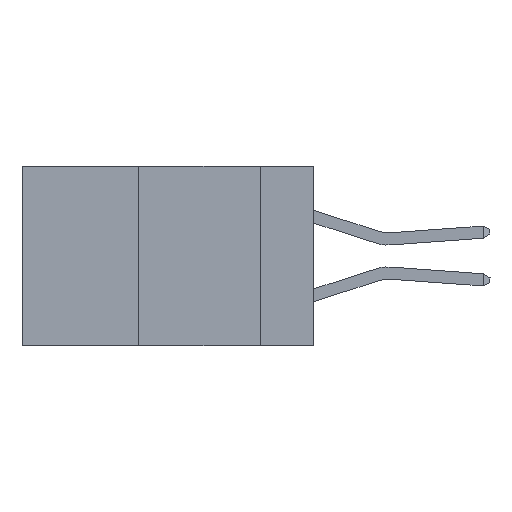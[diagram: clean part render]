
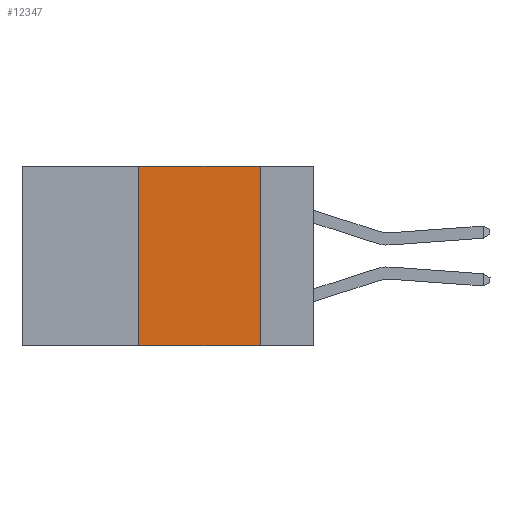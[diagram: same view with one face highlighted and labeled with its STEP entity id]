
A CAD part, left-side view. The second image highlights one B-rep face of the part: STEP entity #12347.
In plain terms, the highlighted planar face has unit normal (-1, 0, 0).
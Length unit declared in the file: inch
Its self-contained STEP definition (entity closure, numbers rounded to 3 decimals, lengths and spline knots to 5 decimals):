
#113 = DIRECTION ( 'NONE',  ( 0., 0., -1. ) ) ;
#137 = LINE ( 'NONE', #12398, #3950 ) ;
#173 = ORIENTED_EDGE ( 'NONE', *, *, #17233, .T. ) ;
#1226 = ORIENTED_EDGE ( 'NONE', *, *, #10822, .F. ) ;
#2858 = EDGE_LOOP ( 'NONE', ( #1226, #11848, #3285, #173 ) ) ;
#3285 = ORIENTED_EDGE ( 'NONE', *, *, #15034, .F. ) ;
#3747 = CARTESIAN_POINT ( 'NONE',  ( 0., 0.11, -0.37 ) ) ;
#3950 = VECTOR ( 'NONE', #15524, 39.37008 ) ;
#5237 = DIRECTION ( 'NONE',  ( 0., 0., 1. ) ) ;
#5273 = VERTEX_POINT ( 'NONE', #16228 ) ;
#5335 = VERTEX_POINT ( 'NONE', #11911 ) ;
#5646 = LINE ( 'NONE', #10524, #16521 ) ;
#5786 = DIRECTION ( 'NONE',  ( 0., 0., -1. ) ) ;
#6332 = VERTEX_POINT ( 'NONE', #3747 ) ;
#7597 = CARTESIAN_POINT ( 'NONE',  ( 0., 0.6, 0. ) ) ;
#9535 = LINE ( 'NONE', #7597, #13103 ) ;
#9648 = EDGE_CURVE ( 'NONE', #5273, #5335, #9535, .T. ) ;
#10524 = CARTESIAN_POINT ( 'NONE',  ( 0., 0.11, 0. ) ) ;
#10822 = EDGE_CURVE ( 'NONE', #5335, #6332, #5646, .T. ) ;
#11848 = ORIENTED_EDGE ( 'NONE', *, *, #9648, .F. ) ;
#11911 = CARTESIAN_POINT ( 'NONE',  ( 0., 0.11, 0. ) ) ;
#12039 = DIRECTION ( 'NONE',  ( 0., -1., 0. ) ) ;
#12243 = CARTESIAN_POINT ( 'NONE',  ( 0., 0.36, -0.37 ) ) ;
#12347 = ADVANCED_FACE ( 'NONE', ( #13664 ), #13435, .F. ) ;
#12398 = CARTESIAN_POINT ( 'NONE',  ( 0., 0.6, -0.37 ) ) ;
#13103 = VECTOR ( 'NONE', #12039, 39.37008 ) ;
#13435 = PLANE ( 'NONE',  #16204 ) ;
#13664 = FACE_OUTER_BOUND ( 'NONE', #2858, .T. ) ;
#14464 = VERTEX_POINT ( 'NONE', #12243 ) ;
#14915 = VECTOR ( 'NONE', #5237, 39.37008 ) ;
#14919 = CARTESIAN_POINT ( 'NONE',  ( 0., 0.6, 0. ) ) ;
#15034 = EDGE_CURVE ( 'NONE', #14464, #5273, #19325, .T. ) ;
#15357 = DIRECTION ( 'NONE',  ( 1., 0., 0. ) ) ;
#15524 = DIRECTION ( 'NONE',  ( 0., -1., 0. ) ) ;
#16204 = AXIS2_PLACEMENT_3D ( 'NONE', #14919, #15357, #113 ) ;
#16228 = CARTESIAN_POINT ( 'NONE',  ( 0., 0.36, 0. ) ) ;
#16521 = VECTOR ( 'NONE', #5786, 39.37008 ) ;
#17233 = EDGE_CURVE ( 'NONE', #14464, #6332, #137, .T. ) ;
#18877 = CARTESIAN_POINT ( 'NONE',  ( 0., 0.36, 0. ) ) ;
#19325 = LINE ( 'NONE', #18877, #14915 ) ;
